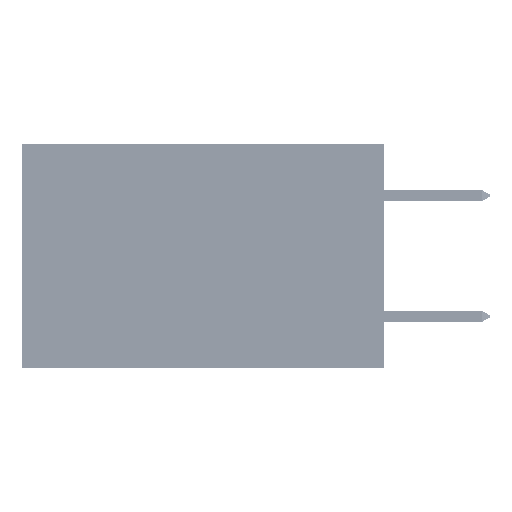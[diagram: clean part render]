
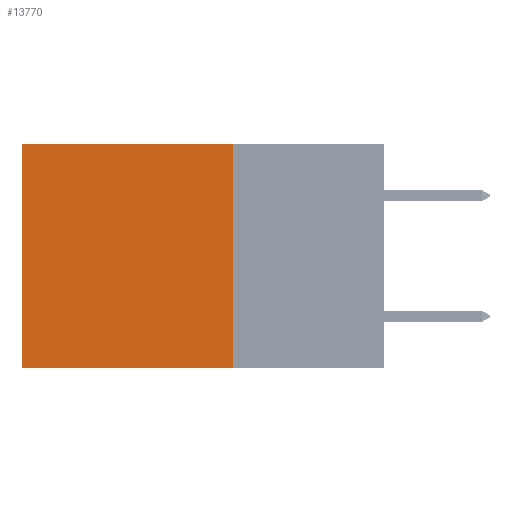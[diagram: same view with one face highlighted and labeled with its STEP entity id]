
A CAD part, left-side view. The second image highlights one B-rep face of the part: STEP entity #13770.
In plain terms, the highlighted planar face has unit normal (-1, 0, 0).
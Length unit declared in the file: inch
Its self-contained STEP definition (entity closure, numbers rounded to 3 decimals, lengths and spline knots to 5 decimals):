
#284 = CARTESIAN_POINT ( 'NONE',  ( 0.2875, 0.25, -0.37 ) ) ;
#592 = CARTESIAN_POINT ( 'NONE',  ( 0.2875, 0.25, 0. ) ) ;
#623 = DIRECTION ( 'NONE',  ( 0., 1., 0. ) ) ;
#1535 = CARTESIAN_POINT ( 'NONE',  ( 0.2875, 0.25, 0. ) ) ;
#2239 = DIRECTION ( 'NONE',  ( 0., 1., 0. ) ) ;
#2597 = DIRECTION ( 'NONE',  ( 0., 0., -1. ) ) ;
#2754 = ORIENTED_EDGE ( 'NONE', *, *, #34678, .F. ) ;
#3356 = EDGE_LOOP ( 'NONE', ( #33840, #2754, #19350, #12983 ) ) ;
#3851 = EDGE_CURVE ( 'NONE', #44461, #14892, #29850, .T. ) ;
#8623 = PLANE ( 'NONE',  #37218 ) ;
#12983 = ORIENTED_EDGE ( 'NONE', *, *, #32421, .T. ) ;
#13770 = ADVANCED_FACE ( 'NONE', ( #38524 ), #8623, .F. ) ;
#14269 = LINE ( 'NONE', #284, #23396 ) ;
#14892 = VERTEX_POINT ( 'NONE', #28576 ) ;
#19350 = ORIENTED_EDGE ( 'NONE', *, *, #3851, .F. ) ;
#21983 = VECTOR ( 'NONE', #41968, 39.37008 ) ;
#22498 = CARTESIAN_POINT ( 'NONE',  ( 0.2875, 0.6, 0. ) ) ;
#23396 = VECTOR ( 'NONE', #623, 39.37008 ) ;
#23566 = VECTOR ( 'NONE', #2239, 39.37008 ) ;
#28082 = EDGE_CURVE ( 'NONE', #38072, #47191, #48278, .T. ) ;
#28576 = CARTESIAN_POINT ( 'NONE',  ( 0.2875, 0.25, -0.37 ) ) ;
#29850 = LINE ( 'NONE', #41532, #32305 ) ;
#32305 = VECTOR ( 'NONE', #2597, 39.37008 ) ;
#32421 = EDGE_CURVE ( 'NONE', #44461, #38072, #33970, .T. ) ;
#33840 = ORIENTED_EDGE ( 'NONE', *, *, #28082, .T. ) ;
#33970 = LINE ( 'NONE', #45645, #23566 ) ;
#34678 = EDGE_CURVE ( 'NONE', #14892, #47191, #14269, .T. ) ;
#35959 = DIRECTION ( 'NONE',  ( 1., 0., 0. ) ) ;
#37218 = AXIS2_PLACEMENT_3D ( 'NONE', #592, #35959, #47928 ) ;
#38072 = VERTEX_POINT ( 'NONE', #43885 ) ;
#38524 = FACE_OUTER_BOUND ( 'NONE', #3356, .T. ) ;
#41532 = CARTESIAN_POINT ( 'NONE',  ( 0.2875, 0.25, 0. ) ) ;
#41968 = DIRECTION ( 'NONE',  ( 0., 0., -1. ) ) ;
#43885 = CARTESIAN_POINT ( 'NONE',  ( 0.2875, 0.6, 0. ) ) ;
#44461 = VERTEX_POINT ( 'NONE', #1535 ) ;
#45645 = CARTESIAN_POINT ( 'NONE',  ( 0.2875, 0.25, 0. ) ) ;
#46692 = CARTESIAN_POINT ( 'NONE',  ( 0.2875, 0.6, -0.37 ) ) ;
#47191 = VERTEX_POINT ( 'NONE', #46692 ) ;
#47928 = DIRECTION ( 'NONE',  ( 0., 0., -1. ) ) ;
#48278 = LINE ( 'NONE', #22498, #21983 ) ;
